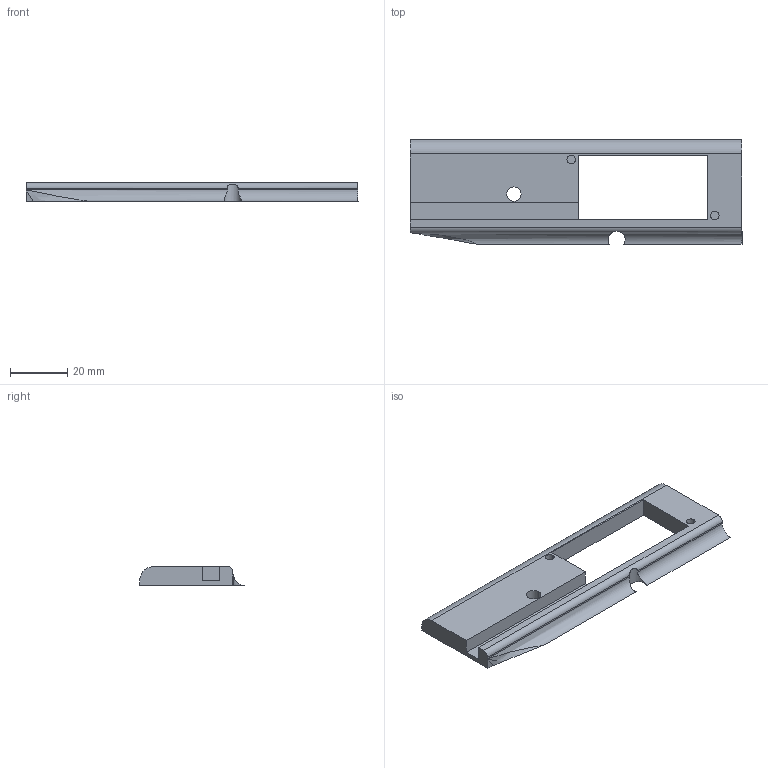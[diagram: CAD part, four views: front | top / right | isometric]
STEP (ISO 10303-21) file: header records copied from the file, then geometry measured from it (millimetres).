
FILE_DESCRIPTION (( 'STEP AP214' ), '1' );
FILE_NAME ('Receiver_Forward_Panel_Right_2.step', '2014-05-14T06:10:11', ( 'WarFairy' ), ( '' ), 'SwSTEP 2.0', 'SolidWorks 2013', '' );
FILE_SCHEMA (( 'AUTOMOTIVE_DESIGN' ));
Length unit declared in the file: inch
Products named in the file (1): Receiver_Forward_Panel_Right_2
Bounding box: 115.7 x 36.5 x 6.57 mm (x, y, z)
Volume: 15711.5 mm3; surface area: 9266.2 mm2
Topology: 1 solids, 1 shells, 30 faces, 80 edges, 52 vertices
Faces by surface type: plane 15, cylinder 14, bspline 1
Entity records: 1245 total; most frequent: CARTESIAN_POINT 451, ORIENTED_EDGE 158, DIRECTION 152, EDGE_CURVE 79, VERTEX_POINT 52, AXIS2_PLACEMENT_3D 51, VECTOR 50, LINE 50
